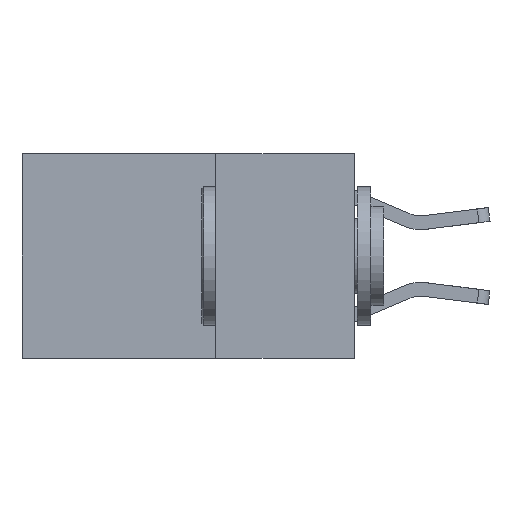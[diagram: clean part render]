
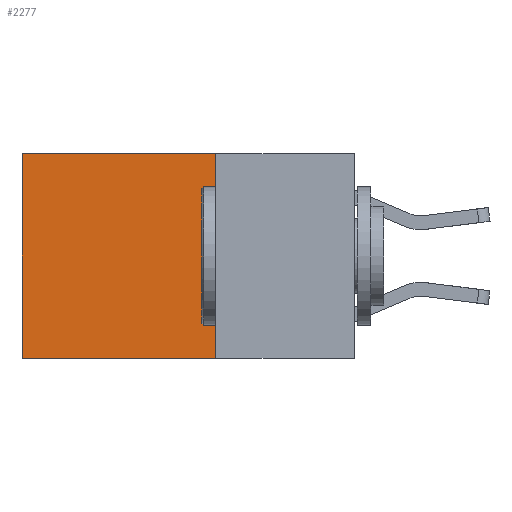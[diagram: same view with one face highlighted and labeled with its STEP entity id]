
A CAD part, left-side view. The second image highlights one B-rep face of the part: STEP entity #2277.
In plain terms, the highlighted planar face has unit normal (-1, 0, 0).
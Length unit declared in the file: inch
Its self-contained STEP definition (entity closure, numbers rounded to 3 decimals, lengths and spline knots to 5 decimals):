
#110 = DIRECTION ( 'NONE',  ( 0., 1., 0. ) ) ;
#478 = VECTOR ( 'NONE', #110, 39.37008 ) ;
#582 = EDGE_CURVE ( 'NONE', #3351, #3657, #9090, .T. ) ;
#939 = CARTESIAN_POINT ( 'NONE',  ( 0.2625, 0.25, -0.37 ) ) ;
#940 = FACE_OUTER_BOUND ( 'NONE', #3221, .T. ) ;
#1300 = LINE ( 'NONE', #9345, #6155 ) ;
#2277 = ADVANCED_FACE ( 'NONE', ( #940 ), #3039, .F. ) ;
#2733 = DIRECTION ( 'NONE',  ( 0., 0., -1. ) ) ;
#2765 = DIRECTION ( 'NONE',  ( 1., 0., 0. ) ) ;
#2769 = CARTESIAN_POINT ( 'NONE',  ( 0.2625, 0.25, 0. ) ) ;
#2830 = CARTESIAN_POINT ( 'NONE',  ( 0.2625, 0.25, 0. ) ) ;
#3039 = PLANE ( 'NONE',  #7236 ) ;
#3200 = DIRECTION ( 'NONE',  ( 0., 0., -1. ) ) ;
#3221 = EDGE_LOOP ( 'NONE', ( #7237, #7251, #7448, #7456 ) ) ;
#3351 = VERTEX_POINT ( 'NONE', #2769 ) ;
#3368 = VECTOR ( 'NONE', #4900, 39.37008 ) ;
#3564 = EDGE_CURVE ( 'NONE', #3657, #5024, #1300, .T. ) ;
#3657 = VERTEX_POINT ( 'NONE', #5079 ) ;
#3951 = CARTESIAN_POINT ( 'NONE',  ( 0.2625, 0.25, 0. ) ) ;
#4021 = CARTESIAN_POINT ( 'NONE',  ( 0.2625, 0.25, 0. ) ) ;
#4408 = VECTOR ( 'NONE', #9078, 39.37008 ) ;
#4900 = DIRECTION ( 'NONE',  ( 0., 0., -1. ) ) ;
#5010 = LINE ( 'NONE', #939, #478 ) ;
#5024 = VERTEX_POINT ( 'NONE', #5248 ) ;
#5079 = CARTESIAN_POINT ( 'NONE',  ( 0.2625, 0.6, 0. ) ) ;
#5248 = CARTESIAN_POINT ( 'NONE',  ( 0.2625, 0.6, -0.37 ) ) ;
#6155 = VECTOR ( 'NONE', #3200, 39.37008 ) ;
#7236 = AXIS2_PLACEMENT_3D ( 'NONE', #2830, #2765, #2733 ) ;
#7237 = ORIENTED_EDGE ( 'NONE', *, *, #3564, .T. ) ;
#7251 = ORIENTED_EDGE ( 'NONE', *, *, #10751, .F. ) ;
#7448 = ORIENTED_EDGE ( 'NONE', *, *, #9339, .F. ) ;
#7456 = ORIENTED_EDGE ( 'NONE', *, *, #582, .T. ) ;
#8599 = LINE ( 'NONE', #3951, #3368 ) ;
#8947 = VERTEX_POINT ( 'NONE', #10383 ) ;
#9078 = DIRECTION ( 'NONE',  ( 0., 1., 0. ) ) ;
#9090 = LINE ( 'NONE', #4021, #4408 ) ;
#9339 = EDGE_CURVE ( 'NONE', #3351, #8947, #8599, .T. ) ;
#9345 = CARTESIAN_POINT ( 'NONE',  ( 0.2625, 0.6, 0. ) ) ;
#10383 = CARTESIAN_POINT ( 'NONE',  ( 0.2625, 0.25, -0.37 ) ) ;
#10751 = EDGE_CURVE ( 'NONE', #8947, #5024, #5010, .T. ) ;
